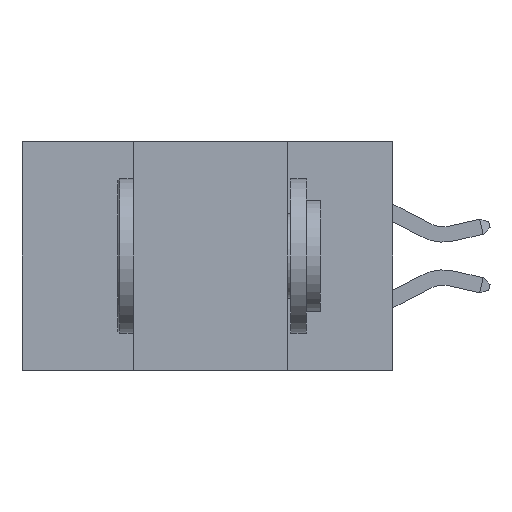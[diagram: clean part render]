
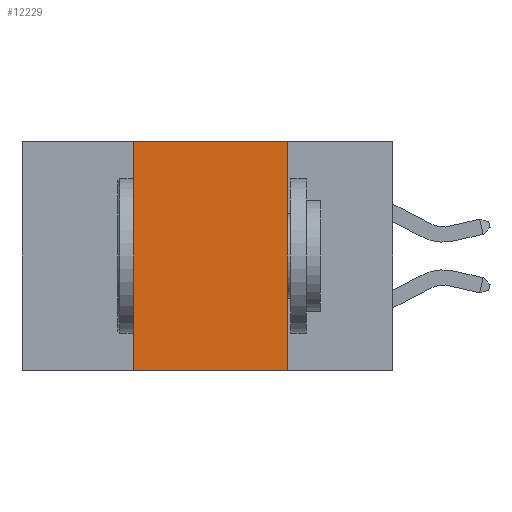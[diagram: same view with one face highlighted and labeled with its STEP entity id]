
A CAD part, left-side view. The second image highlights one B-rep face of the part: STEP entity #12229.
In plain terms, the highlighted planar face has unit normal (-1, 0, 0).
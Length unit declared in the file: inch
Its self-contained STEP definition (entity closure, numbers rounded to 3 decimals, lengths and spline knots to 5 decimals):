
#381 = PLANE ( 'NONE',  #16444 ) ;
#599 = VECTOR ( 'NONE', #9986, 39.37008 ) ;
#1431 = DIRECTION ( 'NONE',  ( 0., 0., 1. ) ) ;
#1699 = EDGE_CURVE ( 'NONE', #1746, #7158, #5876, .T. ) ;
#1746 = VERTEX_POINT ( 'NONE', #9901 ) ;
#1986 = CARTESIAN_POINT ( 'NONE',  ( 0., 0.6, 0. ) ) ;
#2209 = DIRECTION ( 'NONE',  ( 0., -1., 0. ) ) ;
#2982 = VECTOR ( 'NONE', #1431, 39.37008 ) ;
#3622 = ORIENTED_EDGE ( 'NONE', *, *, #16134, .T. ) ;
#3904 = CARTESIAN_POINT ( 'NONE',  ( 0., 0.17, 0. ) ) ;
#3928 = EDGE_CURVE ( 'NONE', #18443, #1746, #4582, .T. ) ;
#4582 = LINE ( 'NONE', #14738, #13815 ) ;
#5023 = DIRECTION ( 'NONE',  ( 0., 0., -1. ) ) ;
#5671 = DIRECTION ( 'NONE',  ( 0., -1., 0. ) ) ;
#5876 = LINE ( 'NONE', #3904, #599 ) ;
#6132 = ORIENTED_EDGE ( 'NONE', *, *, #1699, .F. ) ;
#6842 = VECTOR ( 'NONE', #2209, 39.37008 ) ;
#7158 = VERTEX_POINT ( 'NONE', #12672 ) ;
#7392 = CARTESIAN_POINT ( 'NONE',  ( 0., 0.42, -0.37 ) ) ;
#7970 = CARTESIAN_POINT ( 'NONE',  ( 0., 0.6, -0.37 ) ) ;
#8101 = CARTESIAN_POINT ( 'NONE',  ( 0., 0.42, 0. ) ) ;
#8840 = ORIENTED_EDGE ( 'NONE', *, *, #8871, .F. ) ;
#8871 = EDGE_CURVE ( 'NONE', #17155, #18443, #11283, .T. ) ;
#9901 = CARTESIAN_POINT ( 'NONE',  ( 0., 0.17, 0. ) ) ;
#9986 = DIRECTION ( 'NONE',  ( 0., 0., -1. ) ) ;
#11283 = LINE ( 'NONE', #13046, #2982 ) ;
#12229 = ADVANCED_FACE ( 'NONE', ( #13747 ), #381, .F. ) ;
#12660 = DIRECTION ( 'NONE',  ( 1., 0., 0. ) ) ;
#12672 = CARTESIAN_POINT ( 'NONE',  ( 0., 0.17, -0.37 ) ) ;
#13046 = CARTESIAN_POINT ( 'NONE',  ( 0., 0.42, 0. ) ) ;
#13747 = FACE_OUTER_BOUND ( 'NONE', #18385, .T. ) ;
#13815 = VECTOR ( 'NONE', #5671, 39.37008 ) ;
#14738 = CARTESIAN_POINT ( 'NONE',  ( 0., 0.6, 0. ) ) ;
#14920 = LINE ( 'NONE', #7970, #6842 ) ;
#16134 = EDGE_CURVE ( 'NONE', #17155, #7158, #14920, .T. ) ;
#16444 = AXIS2_PLACEMENT_3D ( 'NONE', #1986, #12660, #5023 ) ;
#17155 = VERTEX_POINT ( 'NONE', #7392 ) ;
#18385 = EDGE_LOOP ( 'NONE', ( #6132, #19559, #8840, #3622 ) ) ;
#18443 = VERTEX_POINT ( 'NONE', #8101 ) ;
#19559 = ORIENTED_EDGE ( 'NONE', *, *, #3928, .F. ) ;
